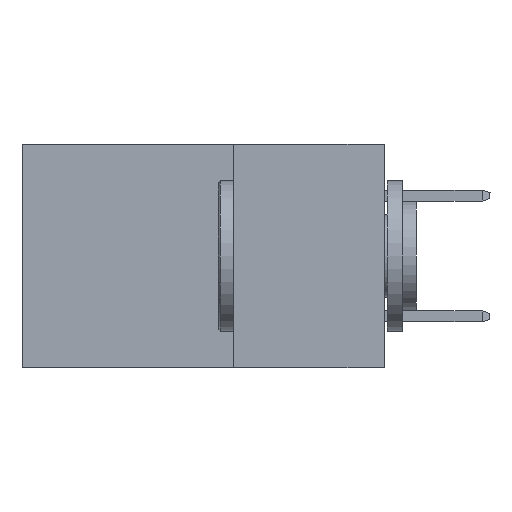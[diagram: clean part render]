
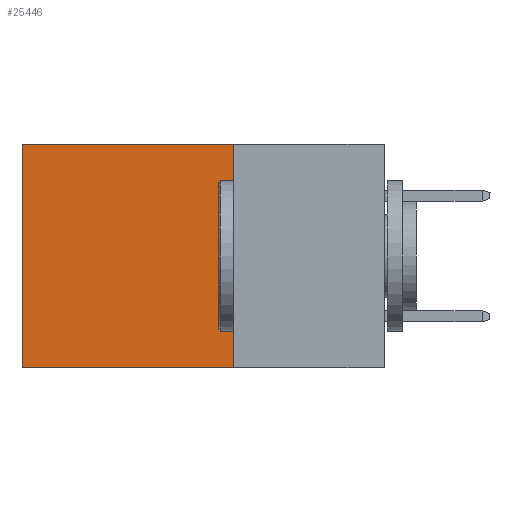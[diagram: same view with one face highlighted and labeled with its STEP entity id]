
A CAD part, left-side view. The second image highlights one B-rep face of the part: STEP entity #25446.
In plain terms, the highlighted planar face has unit normal (-1, 0, 0).
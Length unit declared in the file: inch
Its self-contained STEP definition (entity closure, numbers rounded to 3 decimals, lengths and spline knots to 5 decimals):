
#1669 = VERTEX_POINT ( 'NONE', #26884 ) ;
#2470 = CARTESIAN_POINT ( 'NONE',  ( 0.298, 0.25, 0. ) ) ;
#2627 = PLANE ( 'NONE',  #20488 ) ;
#2820 = DIRECTION ( 'NONE',  ( 1., 0., 0. ) ) ;
#2935 = CARTESIAN_POINT ( 'NONE',  ( 0.298, 0.6, 0. ) ) ;
#3827 = VECTOR ( 'NONE', #27577, 39.37008 ) ;
#4961 = CARTESIAN_POINT ( 'NONE',  ( 0.298, 0.25, 0. ) ) ;
#7207 = DIRECTION ( 'NONE',  ( 0., 0., -1. ) ) ;
#7494 = ORIENTED_EDGE ( 'NONE', *, *, #22668, .T. ) ;
#7906 = LINE ( 'NONE', #8093, #10992 ) ;
#8025 = VERTEX_POINT ( 'NONE', #2470 ) ;
#8093 = CARTESIAN_POINT ( 'NONE',  ( 0.298, 0.25, -0.37 ) ) ;
#9443 = DIRECTION ( 'NONE',  ( 0., 0., -1. ) ) ;
#9615 = DIRECTION ( 'NONE',  ( 0., 0., -1. ) ) ;
#10231 = ORIENTED_EDGE ( 'NONE', *, *, #18733, .F. ) ;
#10513 = LINE ( 'NONE', #11774, #15651 ) ;
#10992 = VECTOR ( 'NONE', #25778, 39.37008 ) ;
#11774 = CARTESIAN_POINT ( 'NONE',  ( 0.298, 0.6, 0. ) ) ;
#11792 = VERTEX_POINT ( 'NONE', #23294 ) ;
#12039 = CARTESIAN_POINT ( 'NONE',  ( 0.298, 0.25, 0. ) ) ;
#12155 = LINE ( 'NONE', #12039, #3827 ) ;
#14173 = VERTEX_POINT ( 'NONE', #2935 ) ;
#14897 = EDGE_CURVE ( 'NONE', #8025, #14173, #12155, .T. ) ;
#15651 = VECTOR ( 'NONE', #7207, 39.37008 ) ;
#16058 = ORIENTED_EDGE ( 'NONE', *, *, #14897, .T. ) ;
#17856 = LINE ( 'NONE', #18419, #21634 ) ;
#18419 = CARTESIAN_POINT ( 'NONE',  ( 0.298, 0.25, 0. ) ) ;
#18733 = EDGE_CURVE ( 'NONE', #8025, #1669, #17856, .T. ) ;
#20079 = FACE_OUTER_BOUND ( 'NONE', #22598, .T. ) ;
#20488 = AXIS2_PLACEMENT_3D ( 'NONE', #4961, #2820, #9443 ) ;
#21634 = VECTOR ( 'NONE', #9615, 39.37008 ) ;
#22593 = ORIENTED_EDGE ( 'NONE', *, *, #25826, .F. ) ;
#22598 = EDGE_LOOP ( 'NONE', ( #7494, #22593, #10231, #16058 ) ) ;
#22668 = EDGE_CURVE ( 'NONE', #14173, #11792, #10513, .T. ) ;
#23294 = CARTESIAN_POINT ( 'NONE',  ( 0.298, 0.6, -0.37 ) ) ;
#25446 = ADVANCED_FACE ( 'NONE', ( #20079 ), #2627, .F. ) ;
#25778 = DIRECTION ( 'NONE',  ( 0., 1., 0. ) ) ;
#25826 = EDGE_CURVE ( 'NONE', #1669, #11792, #7906, .T. ) ;
#26884 = CARTESIAN_POINT ( 'NONE',  ( 0.298, 0.25, -0.37 ) ) ;
#27577 = DIRECTION ( 'NONE',  ( 0., 1., 0. ) ) ;
